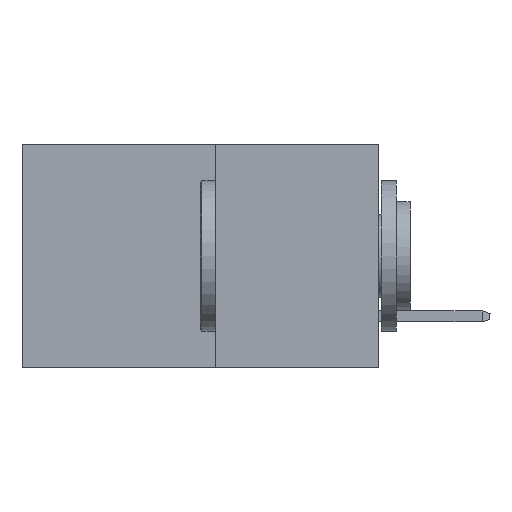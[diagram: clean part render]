
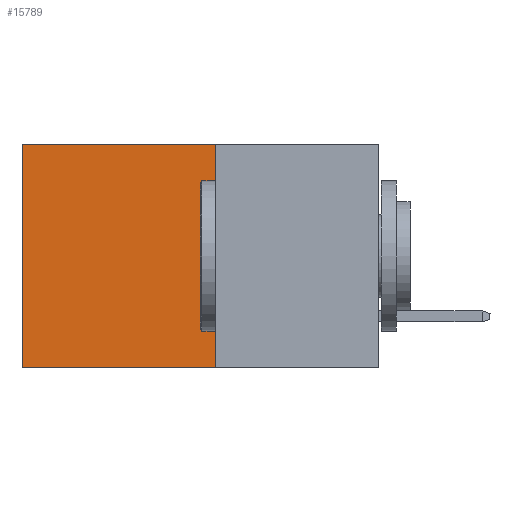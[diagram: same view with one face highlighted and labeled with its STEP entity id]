
A CAD part, left-side view. The second image highlights one B-rep face of the part: STEP entity #15789.
In plain terms, the highlighted planar face has unit normal (-1, 0, 0).
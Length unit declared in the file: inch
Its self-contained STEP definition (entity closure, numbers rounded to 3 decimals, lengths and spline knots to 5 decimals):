
#48 = VECTOR ( 'NONE', #11946, 39.37008 ) ;
#49 = CARTESIAN_POINT ( 'NONE',  ( 0.277, 0.27, -0.37 ) ) ;
#320 = CARTESIAN_POINT ( 'NONE',  ( 0.277, 0.59, -0.37 ) ) ;
#351 = CARTESIAN_POINT ( 'NONE',  ( 0.277, 0.27, 0. ) ) ;
#552 = CARTESIAN_POINT ( 'NONE',  ( 0.277, 0.27, -0.37 ) ) ;
#789 = VERTEX_POINT ( 'NONE', #14939 ) ;
#889 = LINE ( 'NONE', #5056, #10764 ) ;
#1438 = EDGE_CURVE ( 'NONE', #3300, #789, #889, .T. ) ;
#3201 = FACE_OUTER_BOUND ( 'NONE', #13389, .T. ) ;
#3224 = EDGE_CURVE ( 'NONE', #16377, #789, #10301, .T. ) ;
#3300 = VERTEX_POINT ( 'NONE', #9461 ) ;
#4377 = CARTESIAN_POINT ( 'NONE',  ( 0.277, 0.27, 0. ) ) ;
#5011 = DIRECTION ( 'NONE',  ( 0., 1., 0. ) ) ;
#5056 = CARTESIAN_POINT ( 'NONE',  ( 0.277, 0.27, -0.37 ) ) ;
#5710 = DIRECTION ( 'NONE',  ( 1., 0., 0. ) ) ;
#6343 = ORIENTED_EDGE ( 'NONE', *, *, #3224, .T. ) ;
#7920 = CARTESIAN_POINT ( 'NONE',  ( 0.277, 0.59, 0. ) ) ;
#9461 = CARTESIAN_POINT ( 'NONE',  ( 0.277, 0.27, -0.37 ) ) ;
#9526 = PLANE ( 'NONE',  #15216 ) ;
#9848 = ORIENTED_EDGE ( 'NONE', *, *, #13703, .F. ) ;
#10301 = LINE ( 'NONE', #320, #48 ) ;
#10633 = DIRECTION ( 'NONE',  ( 0., 1., 0. ) ) ;
#10764 = VECTOR ( 'NONE', #5011, 39.37008 ) ;
#10879 = ORIENTED_EDGE ( 'NONE', *, *, #10907, .T. ) ;
#10907 = EDGE_CURVE ( 'NONE', #11011, #16377, #12503, .T. ) ;
#11011 = VERTEX_POINT ( 'NONE', #4377 ) ;
#11645 = DIRECTION ( 'NONE',  ( 0., 0., -1. ) ) ;
#11724 = ORIENTED_EDGE ( 'NONE', *, *, #1438, .F. ) ;
#11946 = DIRECTION ( 'NONE',  ( 0., 0., -1. ) ) ;
#12503 = LINE ( 'NONE', #351, #15523 ) ;
#13389 = EDGE_LOOP ( 'NONE', ( #6343, #11724, #9848, #10879 ) ) ;
#13703 = EDGE_CURVE ( 'NONE', #11011, #3300, #16415, .T. ) ;
#14743 = DIRECTION ( 'NONE',  ( 0., 0., -1. ) ) ;
#14939 = CARTESIAN_POINT ( 'NONE',  ( 0.277, 0.59, -0.37 ) ) ;
#15216 = AXIS2_PLACEMENT_3D ( 'NONE', #552, #5710, #14743 ) ;
#15523 = VECTOR ( 'NONE', #10633, 39.37008 ) ;
#15789 = ADVANCED_FACE ( 'NONE', ( #3201 ), #9526, .F. ) ;
#16029 = VECTOR ( 'NONE', #11645, 39.37008 ) ;
#16377 = VERTEX_POINT ( 'NONE', #7920 ) ;
#16415 = LINE ( 'NONE', #49, #16029 ) ;
